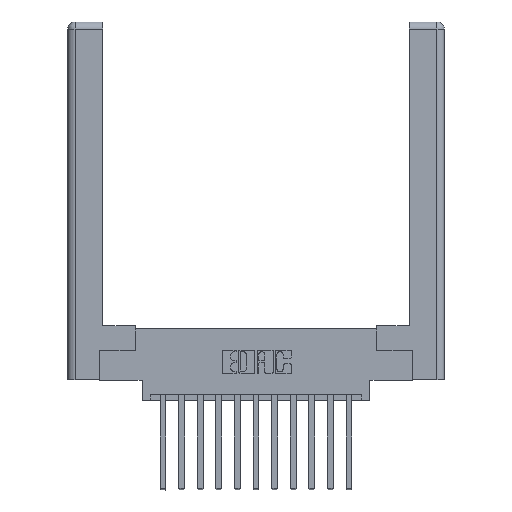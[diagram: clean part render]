
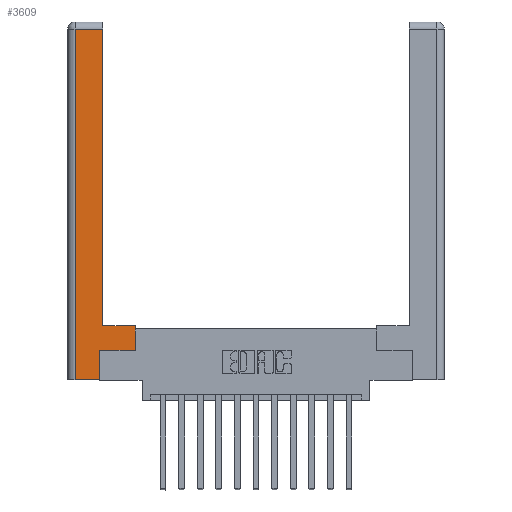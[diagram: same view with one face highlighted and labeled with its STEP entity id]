
A CAD part, top view. The second image highlights one B-rep face of the part: STEP entity #3609.
In plain terms, the highlighted planar face has unit normal (0, 0, 1).
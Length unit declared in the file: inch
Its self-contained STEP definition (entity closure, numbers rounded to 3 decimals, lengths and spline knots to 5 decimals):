
#97 = DIRECTION ( 'NONE',  ( 0., 1., 0. ) ) ;
#314 = ORIENTED_EDGE ( 'NONE', *, *, #6384, .T. ) ;
#532 = DIRECTION ( 'NONE',  ( 0., 1., 0. ) ) ;
#580 = DIRECTION ( 'NONE',  ( 1., 0., 0. ) ) ;
#650 = LINE ( 'NONE', #13016, #3174 ) ;
#651 = EDGE_CURVE ( 'NONE', #7802, #14468, #5896, .T. ) ;
#1686 = DIRECTION ( 'NONE',  ( 0., -1., 0. ) ) ;
#1761 = LINE ( 'NONE', #6787, #9610 ) ;
#2175 = EDGE_CURVE ( 'NONE', #5671, #7802, #14980, .T. ) ;
#2265 = ORIENTED_EDGE ( 'NONE', *, *, #13200, .T. ) ;
#2301 = VECTOR ( 'NONE', #580, 39.37008 ) ;
#2474 = CARTESIAN_POINT ( 'NONE',  ( 0.0615, 2.94, 0. ) ) ;
#2514 = VECTOR ( 'NONE', #10955, 39.37008 ) ;
#3174 = VECTOR ( 'NONE', #10663, 39.37008 ) ;
#3232 = VERTEX_POINT ( 'NONE', #13592 ) ;
#3235 = FACE_OUTER_BOUND ( 'NONE', #10273, .T. ) ;
#3540 = EDGE_CURVE ( 'NONE', #14194, #5515, #5429, .T. ) ;
#3609 = ADVANCED_FACE ( 'NONE', ( #3235 ), #10059, .F. ) ;
#3997 = CARTESIAN_POINT ( 'NONE',  ( 0.0615, 2.94, 0. ) ) ;
#4022 = DIRECTION ( 'NONE',  ( 0., 0., -1. ) ) ;
#4044 = EDGE_CURVE ( 'NONE', #5515, #12385, #5592, .T. ) ;
#4397 = LINE ( 'NONE', #11721, #8797 ) ;
#4439 = ORIENTED_EDGE ( 'NONE', *, *, #12376, .T. ) ;
#4997 = AXIS2_PLACEMENT_3D ( 'NONE', #6461, #4022, #11208 ) ;
#5429 = LINE ( 'NONE', #7436, #2514 ) ;
#5515 = VERTEX_POINT ( 'NONE', #13694 ) ;
#5592 = LINE ( 'NONE', #6316, #2301 ) ;
#5671 = VERTEX_POINT ( 'NONE', #11188 ) ;
#5896 = LINE ( 'NONE', #7630, #8793 ) ;
#6316 = CARTESIAN_POINT ( 'NONE',  ( 0.565, 0.245, 0. ) ) ;
#6371 = LINE ( 'NONE', #7545, #13503 ) ;
#6384 = EDGE_CURVE ( 'NONE', #11459, #5671, #4397, .T. ) ;
#6428 = ORIENTED_EDGE ( 'NONE', *, *, #2175, .T. ) ;
#6461 = CARTESIAN_POINT ( 'NONE',  ( 0., 0., 0. ) ) ;
#6787 = CARTESIAN_POINT ( 'NONE',  ( 0.265, 0., 0. ) ) ;
#7211 = ORIENTED_EDGE ( 'NONE', *, *, #3540, .T. ) ;
#7436 = CARTESIAN_POINT ( 'NONE',  ( 0.265, 0.245, 0. ) ) ;
#7545 = CARTESIAN_POINT ( 'NONE',  ( 0.565, 0.45, 0. ) ) ;
#7630 = CARTESIAN_POINT ( 'NONE',  ( 0.0615, 0., 0. ) ) ;
#7802 = VERTEX_POINT ( 'NONE', #2474 ) ;
#8040 = VECTOR ( 'NONE', #9916, 39.37008 ) ;
#8056 = CARTESIAN_POINT ( 'NONE',  ( 0.295, 0.45, 0. ) ) ;
#8793 = VECTOR ( 'NONE', #1686, 39.37008 ) ;
#8797 = VECTOR ( 'NONE', #97, 39.37008 ) ;
#9315 = DIRECTION ( 'NONE',  ( 1., 0., 0. ) ) ;
#9610 = VECTOR ( 'NONE', #9315, 39.37008 ) ;
#9916 = DIRECTION ( 'NONE',  ( -1., 0., 0. ) ) ;
#10059 = PLANE ( 'NONE',  #4997 ) ;
#10273 = EDGE_LOOP ( 'NONE', ( #314, #6428, #11588, #4439, #7211, #11605, #10868, #2265 ) ) ;
#10663 = DIRECTION ( 'NONE',  ( -1., 0., 0. ) ) ;
#10868 = ORIENTED_EDGE ( 'NONE', *, *, #11700, .T. ) ;
#10955 = DIRECTION ( 'NONE',  ( 0., 1., 0. ) ) ;
#11188 = CARTESIAN_POINT ( 'NONE',  ( 0.295, 2.94, 0. ) ) ;
#11208 = DIRECTION ( 'NONE',  ( -1., 0., 0. ) ) ;
#11459 = VERTEX_POINT ( 'NONE', #8056 ) ;
#11588 = ORIENTED_EDGE ( 'NONE', *, *, #651, .T. ) ;
#11605 = ORIENTED_EDGE ( 'NONE', *, *, #4044, .T. ) ;
#11700 = EDGE_CURVE ( 'NONE', #12385, #3232, #6371, .T. ) ;
#11721 = CARTESIAN_POINT ( 'NONE',  ( 0.295, 3., 0. ) ) ;
#12376 = EDGE_CURVE ( 'NONE', #14468, #14194, #1761, .T. ) ;
#12385 = VERTEX_POINT ( 'NONE', #15092 ) ;
#12892 = CARTESIAN_POINT ( 'NONE',  ( 0.265, 0., 0. ) ) ;
#13016 = CARTESIAN_POINT ( 'NONE',  ( 0.295, 0.45, 0. ) ) ;
#13200 = EDGE_CURVE ( 'NONE', #3232, #11459, #650, .T. ) ;
#13440 = CARTESIAN_POINT ( 'NONE',  ( 0.0615, 0., 0. ) ) ;
#13503 = VECTOR ( 'NONE', #532, 39.37008 ) ;
#13592 = CARTESIAN_POINT ( 'NONE',  ( 0.565, 0.45, 0. ) ) ;
#13694 = CARTESIAN_POINT ( 'NONE',  ( 0.265, 0.245, 0. ) ) ;
#14194 = VERTEX_POINT ( 'NONE', #12892 ) ;
#14468 = VERTEX_POINT ( 'NONE', #13440 ) ;
#14980 = LINE ( 'NONE', #3997, #8040 ) ;
#15092 = CARTESIAN_POINT ( 'NONE',  ( 0.565, 0.245, 0. ) ) ;
